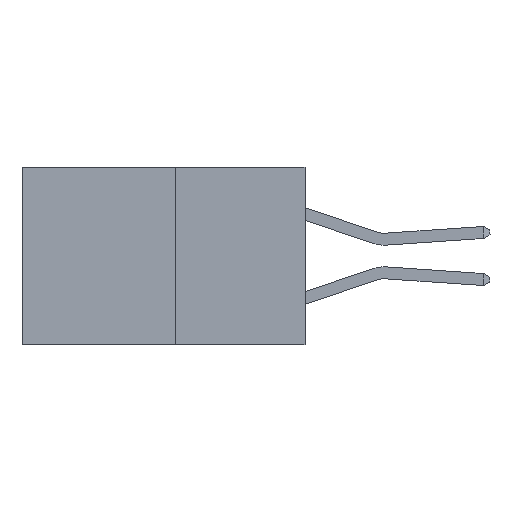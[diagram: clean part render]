
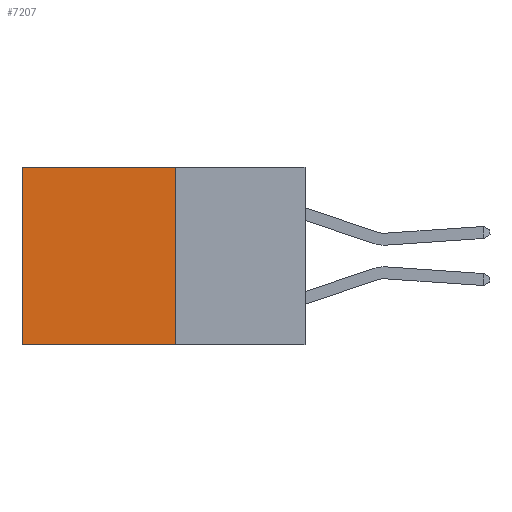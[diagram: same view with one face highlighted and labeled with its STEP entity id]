
A CAD part, left-side view. The second image highlights one B-rep face of the part: STEP entity #7207.
In plain terms, the highlighted planar face has unit normal (-1, 0, 0).
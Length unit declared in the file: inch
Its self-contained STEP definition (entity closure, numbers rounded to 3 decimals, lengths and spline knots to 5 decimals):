
#46 = CARTESIAN_POINT ( 'NONE',  ( 0.277, 0.27, -0.37 ) ) ;
#452 = CARTESIAN_POINT ( 'NONE',  ( 0.277, 0.27, 0. ) ) ;
#580 = EDGE_CURVE ( 'NONE', #3129, #1692, #3310, .T. ) ;
#632 = DIRECTION ( 'NONE',  ( 0., 1., 0. ) ) ;
#834 = VECTOR ( 'NONE', #2149, 39.37008 ) ;
#1039 = CARTESIAN_POINT ( 'NONE',  ( 0.277, 0.59, 0. ) ) ;
#1303 = EDGE_CURVE ( 'NONE', #10367, #7331, #9585, .T. ) ;
#1692 = VERTEX_POINT ( 'NONE', #1039 ) ;
#2122 = EDGE_CURVE ( 'NONE', #1692, #7331, #9455, .T. ) ;
#2133 = DIRECTION ( 'NONE',  ( 0., 1., 0. ) ) ;
#2149 = DIRECTION ( 'NONE',  ( 0., 0., -1. ) ) ;
#2313 = DIRECTION ( 'NONE',  ( 0., 0., -1. ) ) ;
#2426 = CARTESIAN_POINT ( 'NONE',  ( 0.277, 0.59, -0.37 ) ) ;
#2599 = EDGE_CURVE ( 'NONE', #3129, #10367, #2769, .T. ) ;
#2769 = LINE ( 'NONE', #3314, #6809 ) ;
#2791 = CARTESIAN_POINT ( 'NONE',  ( 0.277, 0.27, -0.37 ) ) ;
#2860 = CARTESIAN_POINT ( 'NONE',  ( 0.277, 0.27, 0. ) ) ;
#3114 = DIRECTION ( 'NONE',  ( 0., 0., -1. ) ) ;
#3129 = VERTEX_POINT ( 'NONE', #452 ) ;
#3310 = LINE ( 'NONE', #2860, #9198 ) ;
#3314 = CARTESIAN_POINT ( 'NONE',  ( 0.277, 0.27, -0.37 ) ) ;
#4641 = FACE_OUTER_BOUND ( 'NONE', #4877, .T. ) ;
#4877 = EDGE_LOOP ( 'NONE', ( #6057, #5212, #8152, #6720 ) ) ;
#5212 = ORIENTED_EDGE ( 'NONE', *, *, #1303, .F. ) ;
#5302 = DIRECTION ( 'NONE',  ( 1., 0., 0. ) ) ;
#6057 = ORIENTED_EDGE ( 'NONE', *, *, #2122, .T. ) ;
#6720 = ORIENTED_EDGE ( 'NONE', *, *, #580, .T. ) ;
#6809 = VECTOR ( 'NONE', #2313, 39.37008 ) ;
#6879 = CARTESIAN_POINT ( 'NONE',  ( 0.277, 0.59, -0.37 ) ) ;
#7022 = CARTESIAN_POINT ( 'NONE',  ( 0.277, 0.27, -0.37 ) ) ;
#7184 = PLANE ( 'NONE',  #9784 ) ;
#7207 = ADVANCED_FACE ( 'NONE', ( #4641 ), #7184, .F. ) ;
#7331 = VERTEX_POINT ( 'NONE', #6879 ) ;
#7680 = VECTOR ( 'NONE', #2133, 39.37008 ) ;
#8152 = ORIENTED_EDGE ( 'NONE', *, *, #2599, .F. ) ;
#9198 = VECTOR ( 'NONE', #632, 39.37008 ) ;
#9455 = LINE ( 'NONE', #2426, #834 ) ;
#9585 = LINE ( 'NONE', #46, #7680 ) ;
#9784 = AXIS2_PLACEMENT_3D ( 'NONE', #7022, #5302, #3114 ) ;
#10367 = VERTEX_POINT ( 'NONE', #2791 ) ;
